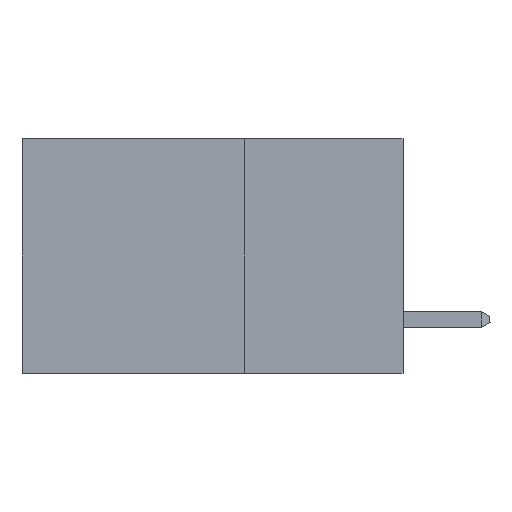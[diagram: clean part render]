
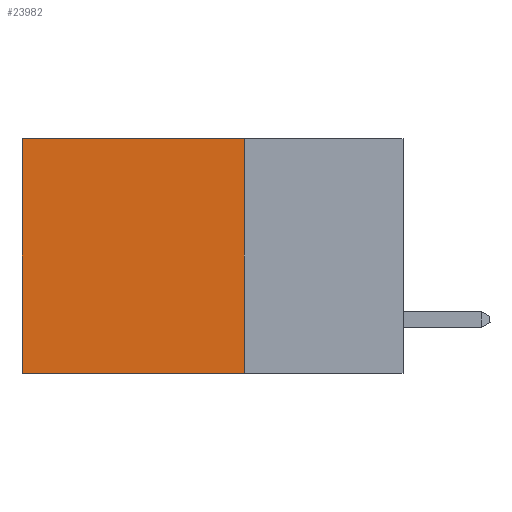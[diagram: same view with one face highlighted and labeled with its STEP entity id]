
A CAD part, left-side view. The second image highlights one B-rep face of the part: STEP entity #23982.
In plain terms, the highlighted planar face has unit normal (-1, 0, 0).
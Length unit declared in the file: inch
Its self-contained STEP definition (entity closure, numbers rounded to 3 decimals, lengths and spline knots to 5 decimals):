
#785 = VERTEX_POINT ( 'NONE', #16793 ) ;
#999 = CARTESIAN_POINT ( 'NONE',  ( 0.2875, 0.25, 0. ) ) ;
#1939 = DIRECTION ( 'NONE',  ( 0., 1., 0. ) ) ;
#2112 = FACE_OUTER_BOUND ( 'NONE', #17499, .T. ) ;
#3994 = ORIENTED_EDGE ( 'NONE', *, *, #9587, .F. ) ;
#4031 = LINE ( 'NONE', #10425, #7776 ) ;
#4237 = AXIS2_PLACEMENT_3D ( 'NONE', #999, #19333, #21362 ) ;
#4293 = ORIENTED_EDGE ( 'NONE', *, *, #14663, .T. ) ;
#4730 = VERTEX_POINT ( 'NONE', #14550 ) ;
#4962 = EDGE_CURVE ( 'NONE', #785, #8202, #5954, .T. ) ;
#5631 = CARTESIAN_POINT ( 'NONE',  ( 0.2875, 0.25, 0. ) ) ;
#5954 = LINE ( 'NONE', #13992, #10350 ) ;
#7776 = VECTOR ( 'NONE', #16835, 39.37008 ) ;
#8202 = VERTEX_POINT ( 'NONE', #16996 ) ;
#9587 = EDGE_CURVE ( 'NONE', #11794, #785, #21975, .T. ) ;
#9770 = DIRECTION ( 'NONE',  ( 0., 0., -1. ) ) ;
#10350 = VECTOR ( 'NONE', #1939, 39.37008 ) ;
#10425 = CARTESIAN_POINT ( 'NONE',  ( 0.2875, 0.25, 0. ) ) ;
#11525 = ORIENTED_EDGE ( 'NONE', *, *, #4962, .F. ) ;
#11794 = VERTEX_POINT ( 'NONE', #5631 ) ;
#13947 = CARTESIAN_POINT ( 'NONE',  ( 0.2875, 0.6, 0. ) ) ;
#13992 = CARTESIAN_POINT ( 'NONE',  ( 0.2875, 0.25, -0.37 ) ) ;
#14550 = CARTESIAN_POINT ( 'NONE',  ( 0.2875, 0.6, 0. ) ) ;
#14663 = EDGE_CURVE ( 'NONE', #11794, #4730, #4031, .T. ) ;
#16793 = CARTESIAN_POINT ( 'NONE',  ( 0.2875, 0.25, -0.37 ) ) ;
#16835 = DIRECTION ( 'NONE',  ( 0., 1., 0. ) ) ;
#16996 = CARTESIAN_POINT ( 'NONE',  ( 0.2875, 0.6, -0.37 ) ) ;
#17499 = EDGE_LOOP ( 'NONE', ( #21775, #11525, #3994, #4293 ) ) ;
#18107 = EDGE_CURVE ( 'NONE', #4730, #8202, #22422, .T. ) ;
#19144 = PLANE ( 'NONE',  #4237 ) ;
#19333 = DIRECTION ( 'NONE',  ( 1., 0., 0. ) ) ;
#21362 = DIRECTION ( 'NONE',  ( 0., 0., -1. ) ) ;
#21513 = VECTOR ( 'NONE', #9770, 39.37008 ) ;
#21775 = ORIENTED_EDGE ( 'NONE', *, *, #18107, .T. ) ;
#21907 = DIRECTION ( 'NONE',  ( 0., 0., -1. ) ) ;
#21975 = LINE ( 'NONE', #22233, #23828 ) ;
#22233 = CARTESIAN_POINT ( 'NONE',  ( 0.2875, 0.25, 0. ) ) ;
#22422 = LINE ( 'NONE', #13947, #21513 ) ;
#23828 = VECTOR ( 'NONE', #21907, 39.37008 ) ;
#23982 = ADVANCED_FACE ( 'NONE', ( #2112 ), #19144, .F. ) ;
